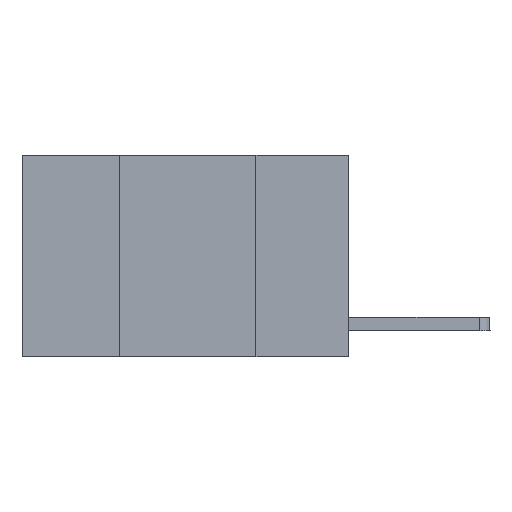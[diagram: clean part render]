
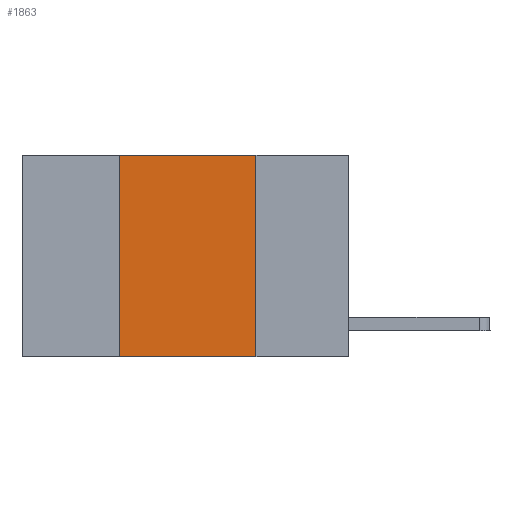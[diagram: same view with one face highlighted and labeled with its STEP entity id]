
A CAD part, left-side view. The second image highlights one B-rep face of the part: STEP entity #1863.
In plain terms, the highlighted planar face has unit normal (-1, 0, 0).
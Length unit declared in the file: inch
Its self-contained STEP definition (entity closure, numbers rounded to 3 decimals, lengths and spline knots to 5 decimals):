
#154 = VECTOR ( 'NONE', #4413, 39.37008 ) ;
#483 = CARTESIAN_POINT ( 'NONE',  ( 0., 0.17, 0. ) ) ;
#485 = CARTESIAN_POINT ( 'NONE',  ( 0., 0.6, 0. ) ) ;
#655 = LINE ( 'NONE', #4783, #6542 ) ;
#1212 = VECTOR ( 'NONE', #9496, 39.37008 ) ;
#1221 = LINE ( 'NONE', #2176, #154 ) ;
#1487 = DIRECTION ( 'NONE',  ( 0., -1., 0. ) ) ;
#1724 = ORIENTED_EDGE ( 'NONE', *, *, #7747, .F. ) ;
#1863 = ADVANCED_FACE ( 'NONE', ( #6805 ), #8423, .F. ) ;
#2176 = CARTESIAN_POINT ( 'NONE',  ( 0., 0.42, 0. ) ) ;
#3097 = VECTOR ( 'NONE', #9148, 39.37008 ) ;
#4044 = EDGE_CURVE ( 'NONE', #10051, #4947, #5946, .T. ) ;
#4353 = VERTEX_POINT ( 'NONE', #7807 ) ;
#4413 = DIRECTION ( 'NONE',  ( 0., 0., 1. ) ) ;
#4616 = ORIENTED_EDGE ( 'NONE', *, *, #4044, .T. ) ;
#4783 = CARTESIAN_POINT ( 'NONE',  ( 0., 0.6, 0. ) ) ;
#4896 = LINE ( 'NONE', #8080, #1212 ) ;
#4947 = VERTEX_POINT ( 'NONE', #6322 ) ;
#5223 = CARTESIAN_POINT ( 'NONE',  ( 0., 0.6, -0.37 ) ) ;
#5780 = EDGE_CURVE ( 'NONE', #4353, #6227, #655, .T. ) ;
#5946 = LINE ( 'NONE', #5223, #3097 ) ;
#6168 = DIRECTION ( 'NONE',  ( 1., 0., 0. ) ) ;
#6227 = VERTEX_POINT ( 'NONE', #483 ) ;
#6322 = CARTESIAN_POINT ( 'NONE',  ( 0., 0.17, -0.37 ) ) ;
#6542 = VECTOR ( 'NONE', #1487, 39.37008 ) ;
#6805 = FACE_OUTER_BOUND ( 'NONE', #9443, .T. ) ;
#7038 = EDGE_CURVE ( 'NONE', #6227, #4947, #4896, .T. ) ;
#7747 = EDGE_CURVE ( 'NONE', #10051, #4353, #1221, .T. ) ;
#7807 = CARTESIAN_POINT ( 'NONE',  ( 0., 0.42, 0. ) ) ;
#8080 = CARTESIAN_POINT ( 'NONE',  ( 0., 0.17, 0. ) ) ;
#8423 = PLANE ( 'NONE',  #9119 ) ;
#8611 = CARTESIAN_POINT ( 'NONE',  ( 0., 0.42, -0.37 ) ) ;
#8981 = ORIENTED_EDGE ( 'NONE', *, *, #7038, .F. ) ;
#9119 = AXIS2_PLACEMENT_3D ( 'NONE', #485, #6168, #9366 ) ;
#9148 = DIRECTION ( 'NONE',  ( 0., -1., 0. ) ) ;
#9366 = DIRECTION ( 'NONE',  ( 0., 0., -1. ) ) ;
#9443 = EDGE_LOOP ( 'NONE', ( #8981, #9527, #1724, #4616 ) ) ;
#9496 = DIRECTION ( 'NONE',  ( 0., 0., -1. ) ) ;
#9527 = ORIENTED_EDGE ( 'NONE', *, *, #5780, .F. ) ;
#10051 = VERTEX_POINT ( 'NONE', #8611 ) ;
